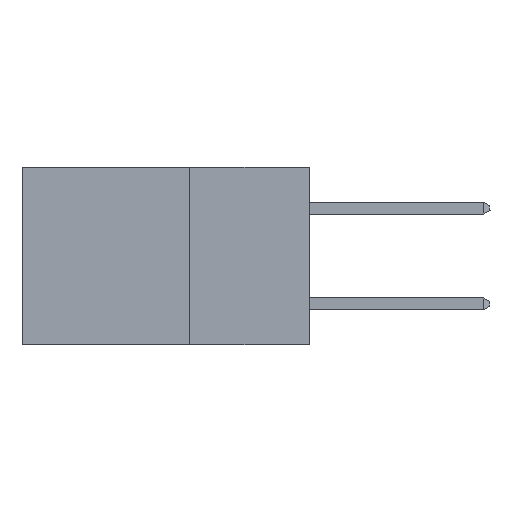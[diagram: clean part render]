
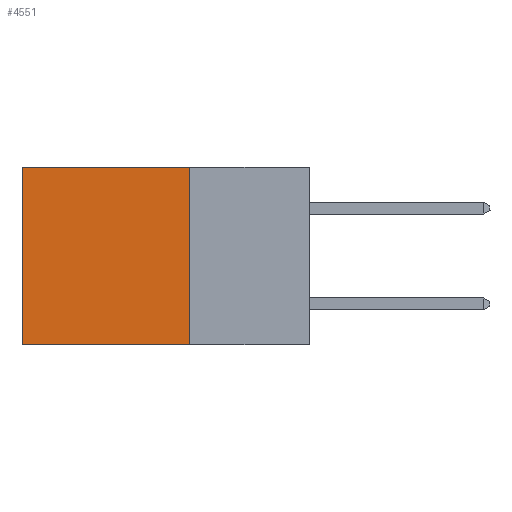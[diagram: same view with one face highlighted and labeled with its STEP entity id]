
A CAD part, left-side view. The second image highlights one B-rep face of the part: STEP entity #4551.
In plain terms, the highlighted planar face has unit normal (-1, 0, 0).
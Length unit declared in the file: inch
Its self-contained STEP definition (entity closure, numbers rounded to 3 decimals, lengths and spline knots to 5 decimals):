
#329 = AXIS2_PLACEMENT_3D ( 'NONE', #5360, #11740, #2768 ) ;
#2488 = DIRECTION ( 'NONE',  ( 0., 1., 0. ) ) ;
#2768 = DIRECTION ( 'NONE',  ( 0., 0., -1. ) ) ;
#3910 = VERTEX_POINT ( 'NONE', #23801 ) ;
#4551 = ADVANCED_FACE ( 'NONE', ( #15313 ), #26866, .F. ) ;
#5360 = CARTESIAN_POINT ( 'NONE',  ( 0.2875, 0.25, 0. ) ) ;
#5926 = CARTESIAN_POINT ( 'NONE',  ( 0.2875, 0.6, 0. ) ) ;
#5942 = CARTESIAN_POINT ( 'NONE',  ( 0.2875, 0.6, -0.37 ) ) ;
#6312 = DIRECTION ( 'NONE',  ( 0., 0., -1. ) ) ;
#8519 = LINE ( 'NONE', #5926, #25042 ) ;
#9482 = LINE ( 'NONE', #15263, #36142 ) ;
#10280 = EDGE_CURVE ( 'NONE', #26294, #23838, #20945, .T. ) ;
#11740 = DIRECTION ( 'NONE',  ( 1., 0., 0. ) ) ;
#14615 = ORIENTED_EDGE ( 'NONE', *, *, #16770, .F. ) ;
#15263 = CARTESIAN_POINT ( 'NONE',  ( 0.2875, 0.25, 0. ) ) ;
#15313 = FACE_OUTER_BOUND ( 'NONE', #22796, .T. ) ;
#16770 = EDGE_CURVE ( 'NONE', #17958, #26294, #9482, .T. ) ;
#17958 = VERTEX_POINT ( 'NONE', #36102 ) ;
#17984 = CARTESIAN_POINT ( 'NONE',  ( 0.2875, 0.25, -0.37 ) ) ;
#18137 = CARTESIAN_POINT ( 'NONE',  ( 0.2875, 0.25, -0.37 ) ) ;
#18531 = ORIENTED_EDGE ( 'NONE', *, *, #25484, .T. ) ;
#20945 = LINE ( 'NONE', #18137, #29781 ) ;
#21389 = LINE ( 'NONE', #27363, #35296 ) ;
#21619 = DIRECTION ( 'NONE',  ( 0., 0., -1. ) ) ;
#22796 = EDGE_LOOP ( 'NONE', ( #18531, #27637, #14615, #33363 ) ) ;
#23733 = DIRECTION ( 'NONE',  ( 0., 1., 0. ) ) ;
#23801 = CARTESIAN_POINT ( 'NONE',  ( 0.2875, 0.6, 0. ) ) ;
#23838 = VERTEX_POINT ( 'NONE', #5942 ) ;
#25042 = VECTOR ( 'NONE', #6312, 39.37008 ) ;
#25484 = EDGE_CURVE ( 'NONE', #3910, #23838, #8519, .T. ) ;
#26294 = VERTEX_POINT ( 'NONE', #17984 ) ;
#26866 = PLANE ( 'NONE',  #329 ) ;
#27363 = CARTESIAN_POINT ( 'NONE',  ( 0.2875, 0.25, 0. ) ) ;
#27637 = ORIENTED_EDGE ( 'NONE', *, *, #10280, .F. ) ;
#29781 = VECTOR ( 'NONE', #23733, 39.37008 ) ;
#29841 = EDGE_CURVE ( 'NONE', #17958, #3910, #21389, .T. ) ;
#33363 = ORIENTED_EDGE ( 'NONE', *, *, #29841, .T. ) ;
#35296 = VECTOR ( 'NONE', #2488, 39.37008 ) ;
#36102 = CARTESIAN_POINT ( 'NONE',  ( 0.2875, 0.25, 0. ) ) ;
#36142 = VECTOR ( 'NONE', #21619, 39.37008 ) ;
